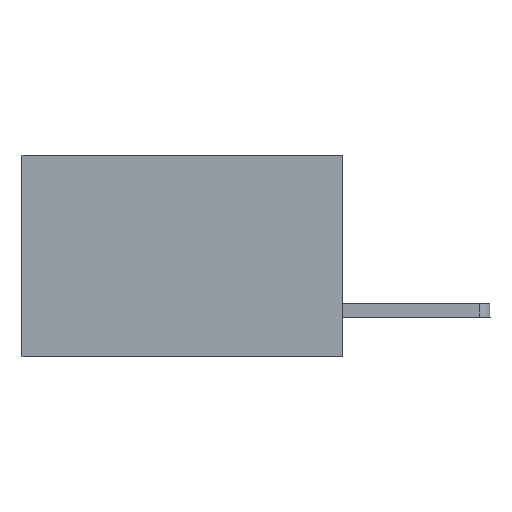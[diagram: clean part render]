
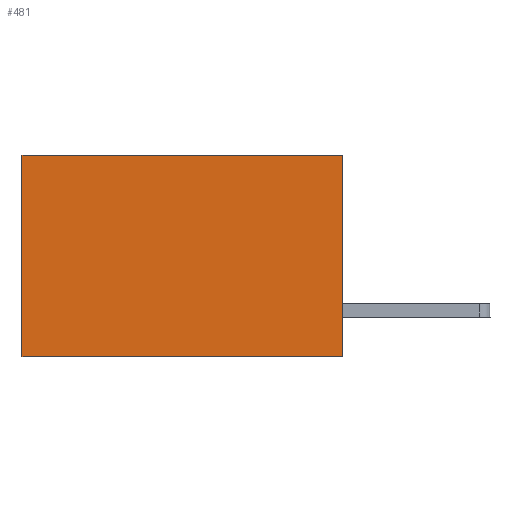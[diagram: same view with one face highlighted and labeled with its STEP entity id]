
A CAD part, left-side view. The second image highlights one B-rep face of the part: STEP entity #481.
In plain terms, the highlighted planar face has unit normal (-1, 0, 0).
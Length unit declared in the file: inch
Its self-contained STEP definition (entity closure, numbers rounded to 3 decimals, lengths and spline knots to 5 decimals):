
#173 = DIRECTION ( 'NONE',  ( 1., 0., 0. ) ) ;
#387 = EDGE_CURVE ( 'NONE', #1478, #8481, #5600, .T. ) ;
#433 = DIRECTION ( 'NONE',  ( 0., 1., 0. ) ) ;
#481 = ADVANCED_FACE ( 'NONE', ( #837 ), #3554, .F. ) ;
#837 = FACE_OUTER_BOUND ( 'NONE', #6789, .T. ) ;
#1010 = DIRECTION ( 'NONE',  ( 0., 0., -1. ) ) ;
#1097 = VERTEX_POINT ( 'NONE', #7658 ) ;
#1295 = EDGE_CURVE ( 'NONE', #1097, #8416, #1802, .T. ) ;
#1478 = VERTEX_POINT ( 'NONE', #1847 ) ;
#1722 = AXIS2_PLACEMENT_3D ( 'NONE', #7029, #173, #4343 ) ;
#1802 = LINE ( 'NONE', #7154, #3292 ) ;
#1847 = CARTESIAN_POINT ( 'NONE',  ( 0.277, 0.59, 0. ) ) ;
#2007 = LINE ( 'NONE', #5085, #8135 ) ;
#2508 = ORIENTED_EDGE ( 'NONE', *, *, #1295, .F. ) ;
#3102 = ORIENTED_EDGE ( 'NONE', *, *, #7358, .T. ) ;
#3286 = VECTOR ( 'NONE', #1010, 39.37008 ) ;
#3292 = VECTOR ( 'NONE', #3762, 39.37008 ) ;
#3554 = PLANE ( 'NONE',  #1722 ) ;
#3762 = DIRECTION ( 'NONE',  ( 0., 0., -1. ) ) ;
#4051 = ORIENTED_EDGE ( 'NONE', *, *, #387, .T. ) ;
#4343 = DIRECTION ( 'NONE',  ( 0., 0., -1. ) ) ;
#4560 = LINE ( 'NONE', #8059, #7890 ) ;
#4714 = DIRECTION ( 'NONE',  ( 0., 1., 0. ) ) ;
#5059 = CARTESIAN_POINT ( 'NONE',  ( 0.277, 0.59, -0.37 ) ) ;
#5085 = CARTESIAN_POINT ( 'NONE',  ( 0.277, 0., -0.37 ) ) ;
#5600 = LINE ( 'NONE', #7625, #3286 ) ;
#6789 = EDGE_LOOP ( 'NONE', ( #4051, #8814, #2508, #3102 ) ) ;
#7029 = CARTESIAN_POINT ( 'NONE',  ( 0.277, 0., -0.37 ) ) ;
#7154 = CARTESIAN_POINT ( 'NONE',  ( 0.277, 0., -0.37 ) ) ;
#7358 = EDGE_CURVE ( 'NONE', #1097, #1478, #4560, .T. ) ;
#7625 = CARTESIAN_POINT ( 'NONE',  ( 0.277, 0.59, -0.37 ) ) ;
#7658 = CARTESIAN_POINT ( 'NONE',  ( 0.277, 0., 0. ) ) ;
#7792 = CARTESIAN_POINT ( 'NONE',  ( 0.277, 0., -0.37 ) ) ;
#7794 = EDGE_CURVE ( 'NONE', #8416, #8481, #2007, .T. ) ;
#7890 = VECTOR ( 'NONE', #433, 39.37008 ) ;
#8059 = CARTESIAN_POINT ( 'NONE',  ( 0.277, 0., 0. ) ) ;
#8135 = VECTOR ( 'NONE', #4714, 39.37008 ) ;
#8416 = VERTEX_POINT ( 'NONE', #7792 ) ;
#8481 = VERTEX_POINT ( 'NONE', #5059 ) ;
#8814 = ORIENTED_EDGE ( 'NONE', *, *, #7794, .F. ) ;
